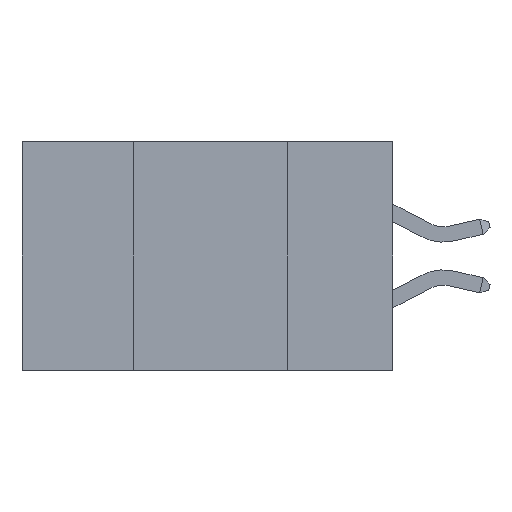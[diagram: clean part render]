
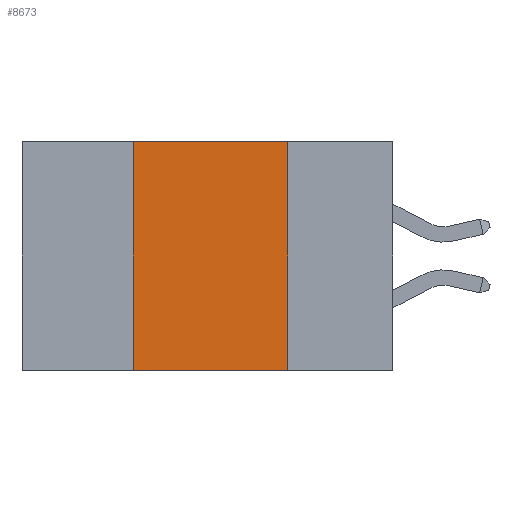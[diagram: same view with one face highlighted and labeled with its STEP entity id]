
A CAD part, left-side view. The second image highlights one B-rep face of the part: STEP entity #8673.
In plain terms, the highlighted planar face has unit normal (-1, 0, 0).
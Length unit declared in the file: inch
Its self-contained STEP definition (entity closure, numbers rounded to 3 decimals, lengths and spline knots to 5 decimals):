
#156 = DIRECTION ( 'NONE',  ( 0., 0., 1. ) ) ;
#315 = EDGE_CURVE ( 'NONE', #7790, #12576, #10707, .T. ) ;
#782 = DIRECTION ( 'NONE',  ( 0., -1., 0. ) ) ;
#788 = CARTESIAN_POINT ( 'NONE',  ( 0., 0.6, 0. ) ) ;
#1122 = CARTESIAN_POINT ( 'NONE',  ( 0., 0.17, 0. ) ) ;
#2727 = DIRECTION ( 'NONE',  ( 0., -1., 0. ) ) ;
#2901 = LINE ( 'NONE', #13707, #10650 ) ;
#3059 = ORIENTED_EDGE ( 'NONE', *, *, #6824, .F. ) ;
#3361 = ORIENTED_EDGE ( 'NONE', *, *, #9455, .T. ) ;
#4810 = CARTESIAN_POINT ( 'NONE',  ( 0., 0.17, 0. ) ) ;
#5104 = VECTOR ( 'NONE', #2727, 39.37008 ) ;
#6689 = AXIS2_PLACEMENT_3D ( 'NONE', #788, #11113, #8190 ) ;
#6711 = LINE ( 'NONE', #1122, #17656 ) ;
#6723 = PLANE ( 'NONE',  #6689 ) ;
#6824 = EDGE_CURVE ( 'NONE', #12576, #13262, #2901, .T. ) ;
#6946 = LINE ( 'NONE', #14274, #5104 ) ;
#7790 = VERTEX_POINT ( 'NONE', #11030 ) ;
#7901 = FACE_OUTER_BOUND ( 'NONE', #15897, .T. ) ;
#8157 = ORIENTED_EDGE ( 'NONE', *, *, #315, .F. ) ;
#8190 = DIRECTION ( 'NONE',  ( 0., 0., -1. ) ) ;
#8673 = ADVANCED_FACE ( 'NONE', ( #7901 ), #6723, .F. ) ;
#9455 = EDGE_CURVE ( 'NONE', #7790, #11517, #6946, .T. ) ;
#10650 = VECTOR ( 'NONE', #782, 39.37008 ) ;
#10707 = LINE ( 'NONE', #17896, #15056 ) ;
#10887 = CARTESIAN_POINT ( 'NONE',  ( 0., 0.42, 0. ) ) ;
#11030 = CARTESIAN_POINT ( 'NONE',  ( 0., 0.42, -0.37 ) ) ;
#11113 = DIRECTION ( 'NONE',  ( 1., 0., 0. ) ) ;
#11517 = VERTEX_POINT ( 'NONE', #18511 ) ;
#12576 = VERTEX_POINT ( 'NONE', #10887 ) ;
#13262 = VERTEX_POINT ( 'NONE', #4810 ) ;
#13707 = CARTESIAN_POINT ( 'NONE',  ( 0., 0.6, 0. ) ) ;
#14267 = DIRECTION ( 'NONE',  ( 0., 0., -1. ) ) ;
#14274 = CARTESIAN_POINT ( 'NONE',  ( 0., 0.6, -0.37 ) ) ;
#15056 = VECTOR ( 'NONE', #156, 39.37008 ) ;
#15090 = ORIENTED_EDGE ( 'NONE', *, *, #16015, .F. ) ;
#15897 = EDGE_LOOP ( 'NONE', ( #15090, #3059, #8157, #3361 ) ) ;
#16015 = EDGE_CURVE ( 'NONE', #13262, #11517, #6711, .T. ) ;
#17656 = VECTOR ( 'NONE', #14267, 39.37008 ) ;
#17896 = CARTESIAN_POINT ( 'NONE',  ( 0., 0.42, 0. ) ) ;
#18511 = CARTESIAN_POINT ( 'NONE',  ( 0., 0.17, -0.37 ) ) ;
